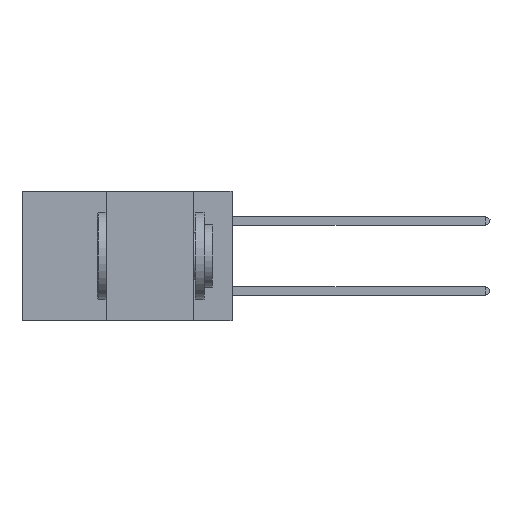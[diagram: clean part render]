
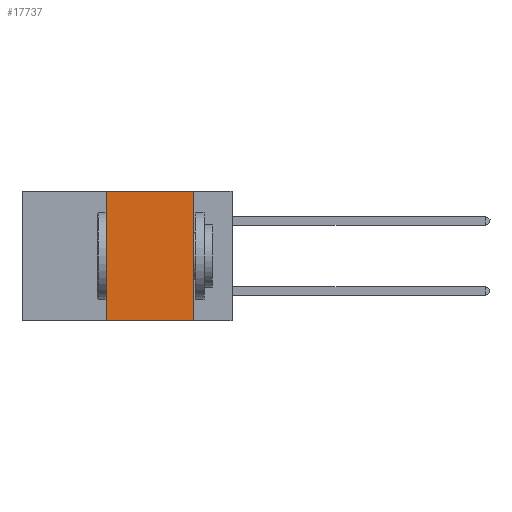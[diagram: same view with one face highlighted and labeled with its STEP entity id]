
A CAD part, left-side view. The second image highlights one B-rep face of the part: STEP entity #17737.
In plain terms, the highlighted planar face has unit normal (-1, 0, 0).
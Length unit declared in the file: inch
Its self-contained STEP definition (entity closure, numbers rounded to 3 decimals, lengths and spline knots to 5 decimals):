
#756 = VERTEX_POINT ( 'NONE', #15417 ) ;
#1453 = EDGE_CURVE ( 'NONE', #12509, #14384, #19617, .T. ) ;
#1509 = ORIENTED_EDGE ( 'NONE', *, *, #25182, .F. ) ;
#2345 = DIRECTION ( 'NONE',  ( 0., 0., -1. ) ) ;
#4963 = LINE ( 'NONE', #17928, #25680 ) ;
#6045 = CARTESIAN_POINT ( 'NONE',  ( 0., 0.6, 0. ) ) ;
#7008 = PLANE ( 'NONE',  #17479 ) ;
#7392 = CARTESIAN_POINT ( 'NONE',  ( 0., 0.11, -0.37 ) ) ;
#7416 = ORIENTED_EDGE ( 'NONE', *, *, #20886, .F. ) ;
#7480 = EDGE_LOOP ( 'NONE', ( #1509, #18409, #7416, #25956 ) ) ;
#8214 = DIRECTION ( 'NONE',  ( 0., 0., -1. ) ) ;
#9074 = EDGE_CURVE ( 'NONE', #18064, #756, #28185, .T. ) ;
#9325 = DIRECTION ( 'NONE',  ( 0., 0., 1. ) ) ;
#9560 = DIRECTION ( 'NONE',  ( 0., -1., 0. ) ) ;
#11358 = DIRECTION ( 'NONE',  ( 1., 0., 0. ) ) ;
#12250 = CARTESIAN_POINT ( 'NONE',  ( 0., 0.6, -0.37 ) ) ;
#12509 = VERTEX_POINT ( 'NONE', #28257 ) ;
#14384 = VERTEX_POINT ( 'NONE', #7392 ) ;
#15104 = VECTOR ( 'NONE', #9560, 39.37008 ) ;
#15417 = CARTESIAN_POINT ( 'NONE',  ( 0., 0.11, 0. ) ) ;
#17479 = AXIS2_PLACEMENT_3D ( 'NONE', #22696, #11358, #2345 ) ;
#17737 = ADVANCED_FACE ( 'NONE', ( #21208 ), #7008, .F. ) ;
#17928 = CARTESIAN_POINT ( 'NONE',  ( 0., 0.36, 0. ) ) ;
#18064 = VERTEX_POINT ( 'NONE', #25483 ) ;
#18409 = ORIENTED_EDGE ( 'NONE', *, *, #9074, .F. ) ;
#19402 = DIRECTION ( 'NONE',  ( 0., -1., 0. ) ) ;
#19617 = LINE ( 'NONE', #12250, #15104 ) ;
#20886 = EDGE_CURVE ( 'NONE', #12509, #18064, #4963, .T. ) ;
#21109 = VECTOR ( 'NONE', #19402, 39.37008 ) ;
#21208 = FACE_OUTER_BOUND ( 'NONE', #7480, .T. ) ;
#21598 = VECTOR ( 'NONE', #8214, 39.37008 ) ;
#22696 = CARTESIAN_POINT ( 'NONE',  ( 0., 0.6, 0. ) ) ;
#25182 = EDGE_CURVE ( 'NONE', #756, #14384, #28978, .T. ) ;
#25483 = CARTESIAN_POINT ( 'NONE',  ( 0., 0.36, 0. ) ) ;
#25680 = VECTOR ( 'NONE', #9325, 39.37008 ) ;
#25956 = ORIENTED_EDGE ( 'NONE', *, *, #1453, .T. ) ;
#28185 = LINE ( 'NONE', #6045, #21109 ) ;
#28257 = CARTESIAN_POINT ( 'NONE',  ( 0., 0.36, -0.37 ) ) ;
#28549 = CARTESIAN_POINT ( 'NONE',  ( 0., 0.11, 0. ) ) ;
#28978 = LINE ( 'NONE', #28549, #21598 ) ;
